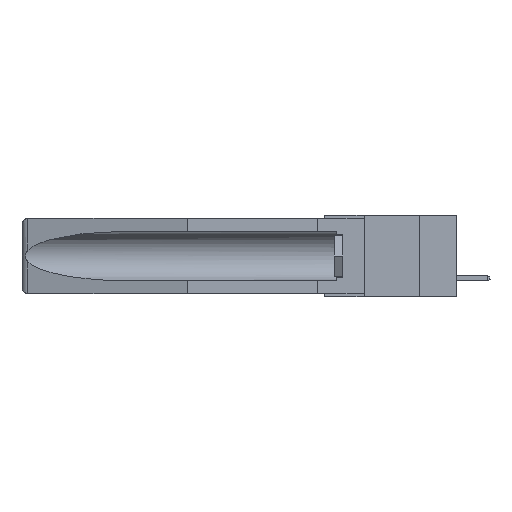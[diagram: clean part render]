
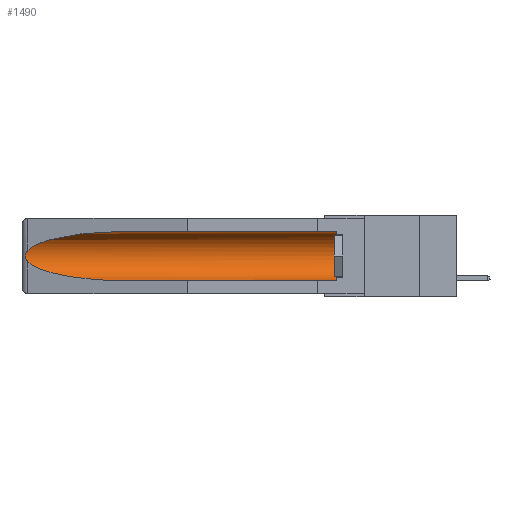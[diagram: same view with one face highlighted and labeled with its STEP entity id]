
A CAD part, left-side view. The second image highlights one B-rep face of the part: STEP entity #1490.
In plain terms, the highlighted cylindrical face has radius 2.857 mm (diameter 5.715 mm), a partial arc.
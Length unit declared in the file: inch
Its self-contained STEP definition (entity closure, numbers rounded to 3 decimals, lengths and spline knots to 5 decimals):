
#868 = EDGE_CURVE ( 'NONE', #18770, #20984, #20541, .T. ) ;
#1475 = CARTESIAN_POINT ( 'NONE',  ( 0.26537, 1.52718, -0.14972 ) ) ;
#1480 = CARTESIAN_POINT ( 'NONE',  ( 0.26537, 1.52718, -0.19328 ) ) ;
#1490 = ADVANCED_FACE ( 'NONE', ( #5688 ), #18795, .F. ) ;
#1741 = CARTESIAN_POINT ( 'NONE',  ( 0.2673, 1.5327, -0.16383 ) ) ;
#2039 = ORIENTED_EDGE ( 'NONE', *, *, #18900, .T. ) ;
#2573 = CARTESIAN_POINT ( 'NONE',  ( 0.155, 0.126, -0.1715 ) ) ;
#2630 = EDGE_CURVE ( 'NONE', #9085, #6043, #18702, .T. ) ;
#3086 = EDGE_CURVE ( 'NONE', #6119, #15734, #8837, .T. ) ;
#3250 = CARTESIAN_POINT ( 'NONE',  ( 0.155, -0.30754, -0.284 ) ) ;
#3514 = ORIENTED_EDGE ( 'NONE', *, *, #2630, .T. ) ;
#3868 = CARTESIAN_POINT ( 'NONE',  ( 0.155, 0.126, -0.059 ) ) ;
#3982 =( BOUNDED_CURVE ( )  B_SPLINE_CURVE ( 3, ( #18063, #12499, #23651, #1475 ),
 .UNSPECIFIED., .F., .F. ) 
 B_SPLINE_CURVE_WITH_KNOTS ( ( 4, 4 ),
 ( 4.71239, 6.08839 ),
 .UNSPECIFIED. ) 
 CURVE ( )  GEOMETRIC_REPRESENTATION_ITEM ( )  RATIONAL_B_SPLINE_CURVE ( ( 1., 0.848, 0.848, 1. ) ) 
 REPRESENTATION_ITEM ( '' )  );
#4290 = VECTOR ( 'NONE', #11561, 39.37008 ) ;
#5688 = FACE_OUTER_BOUND ( 'NONE', #10875, .T. ) ;
#5804 = ORIENTED_EDGE ( 'NONE', *, *, #22248, .T. ) ;
#6043 = VERTEX_POINT ( 'NONE', #17383 ) ;
#6119 = VERTEX_POINT ( 'NONE', #13529 ) ;
#6377 = EDGE_CURVE ( 'NONE', #6043, #15734, #15290, .T. ) ;
#7350 = CARTESIAN_POINT ( 'NONE',  ( 0.26597, 1.52961, -0.15275 ) ) ;
#8015 = CARTESIAN_POINT ( 'NONE',  ( 0.155, -0.30754, -0.1715 ) ) ;
#8837 = LINE ( 'NONE', #3250, #18437 ) ;
#8956 = CARTESIAN_POINT ( 'NONE',  ( 0.25451, 1.48313, -0.24835 ) ) ;
#9085 = VERTEX_POINT ( 'NONE', #9357 ) ;
#9105 = CARTESIAN_POINT ( 'NONE',  ( 0.155, 1.07973, -0.284 ) ) ;
#9116 = CARTESIAN_POINT ( 'NONE',  ( 0.155, 1.07973, -0.284 ) ) ;
#9357 = CARTESIAN_POINT ( 'NONE',  ( 0.26537, 1.52718, -0.14972 ) ) ;
#10649 = CARTESIAN_POINT ( 'NONE',  ( 0.21114, 1.30732, -0.284 ) ) ;
#10747 = CARTESIAN_POINT ( 'NONE',  ( 0.26654, 1.53092, -0.15636 ) ) ;
#10757 = DIRECTION ( 'NONE',  ( 0., 1., 0. ) ) ;
#10821 = CARTESIAN_POINT ( 'NONE',  ( 0.26537, 1.52718, -0.19328 ) ) ;
#10875 = EDGE_LOOP ( 'NONE', ( #5804, #3514, #18071, #12640, #2039, #13157 ) ) ;
#11561 = DIRECTION ( 'NONE',  ( 0., 1., 0. ) ) ;
#12499 = CARTESIAN_POINT ( 'NONE',  ( 0.21114, 1.30732, -0.059 ) ) ;
#12640 = ORIENTED_EDGE ( 'NONE', *, *, #3086, .F. ) ;
#12685 = CARTESIAN_POINT ( 'NONE',  ( 0.2673, 1.53269, -0.17917 ) ) ;
#12755 = AXIS2_PLACEMENT_3D ( 'NONE', #8015, #13593, #15401 ) ;
#13157 = ORIENTED_EDGE ( 'NONE', *, *, #868, .T. ) ;
#13529 = CARTESIAN_POINT ( 'NONE',  ( 0.155, 0.126, -0.284 ) ) ;
#13593 = DIRECTION ( 'NONE',  ( 0., 1., 0. ) ) ;
#14495 = CARTESIAN_POINT ( 'NONE',  ( 0.26655, 1.53094, -0.18657 ) ) ;
#14653 = CARTESIAN_POINT ( 'NONE',  ( 0.2675, 1.53308, -0.16763 ) ) ;
#14734 = CARTESIAN_POINT ( 'NONE',  ( 0.2675, 1.53308, -0.17534 ) ) ;
#14880 = CARTESIAN_POINT ( 'NONE',  ( 0.155, 1.07973, -0.059 ) ) ;
#15290 =( BOUNDED_CURVE ( )  B_SPLINE_CURVE ( 3, ( #1480, #8956, #10649, #9105 ),
 .UNSPECIFIED., .F., .T. ) 
 B_SPLINE_CURVE_WITH_KNOTS ( ( 4, 4 ),
 ( 0.1948, 1.5708 ),
 .UNSPECIFIED. ) 
 CURVE ( )  GEOMETRIC_REPRESENTATION_ITEM ( )  RATIONAL_B_SPLINE_CURVE ( ( 1., 0.848, 0.848, 1. ) ) 
 REPRESENTATION_ITEM ( '' )  );
#15401 = DIRECTION ( 'NONE',  ( 0., 0., 1. ) ) ;
#15481 = DIRECTION ( 'NONE',  ( 0., 0., 1. ) ) ;
#15734 = VERTEX_POINT ( 'NONE', #9116 ) ;
#17108 = CARTESIAN_POINT ( 'NONE',  ( 0.155, -0.30754, -0.059 ) ) ;
#17383 = CARTESIAN_POINT ( 'NONE',  ( 0.26537, 1.52718, -0.19328 ) ) ;
#18063 = CARTESIAN_POINT ( 'NONE',  ( 0.155, 1.07973, -0.059 ) ) ;
#18071 = ORIENTED_EDGE ( 'NONE', *, *, #6377, .T. ) ;
#18437 = VECTOR ( 'NONE', #10757, 39.37008 ) ;
#18702 = B_SPLINE_CURVE_WITH_KNOTS ( 'NONE', 3,
 ( #21845, #7350, #10747, #1741, #14653, #14734, #12685, #14495, #20326, #10821 ),
 .UNSPECIFIED., .F., .F.,
 ( 4, 2, 2, 2, 4 ),
 ( 0., 0.00029, 0.00058, 0.00087, 0.00117 ),
 .UNSPECIFIED. ) ;
#18770 = VERTEX_POINT ( 'NONE', #3868 ) ;
#18795 = CYLINDRICAL_SURFACE ( 'NONE', #12755, 0.1125 ) ;
#18900 = EDGE_CURVE ( 'NONE', #6119, #18770, #20919, .T. ) ;
#20326 = CARTESIAN_POINT ( 'NONE',  ( 0.26597, 1.5296, -0.19026 ) ) ;
#20541 = LINE ( 'NONE', #17108, #4290 ) ;
#20919 = CIRCLE ( 'NONE', #23837, 0.1125 ) ;
#20984 = VERTEX_POINT ( 'NONE', #14880 ) ;
#21127 = DIRECTION ( 'NONE',  ( 0., -1., 0. ) ) ;
#21845 = CARTESIAN_POINT ( 'NONE',  ( 0.26537, 1.52718, -0.14972 ) ) ;
#22248 = EDGE_CURVE ( 'NONE', #20984, #9085, #3982, .T. ) ;
#23651 = CARTESIAN_POINT ( 'NONE',  ( 0.25451, 1.48313, -0.09465 ) ) ;
#23837 = AXIS2_PLACEMENT_3D ( 'NONE', #2573, #21127, #15481 ) ;
